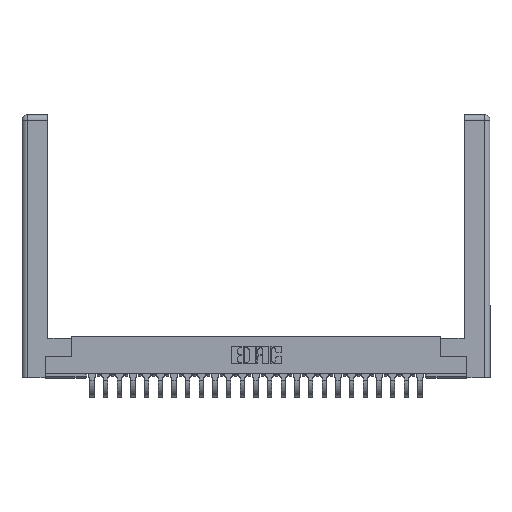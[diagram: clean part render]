
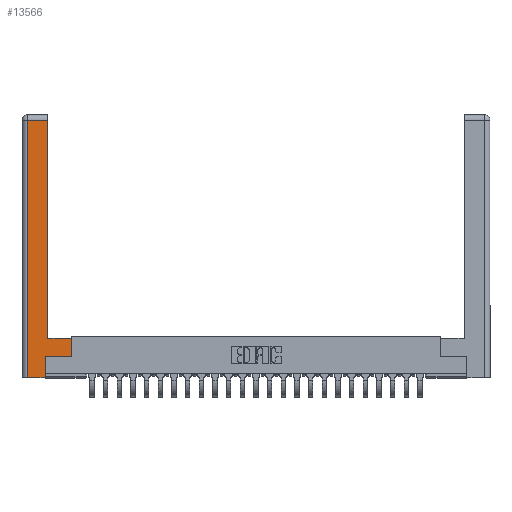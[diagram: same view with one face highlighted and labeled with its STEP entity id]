
A CAD part, top view. The second image highlights one B-rep face of the part: STEP entity #13566.
In plain terms, the highlighted planar face has unit normal (0, 0, 1).
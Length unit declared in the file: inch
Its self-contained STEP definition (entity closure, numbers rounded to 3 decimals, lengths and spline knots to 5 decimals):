
#136 = CARTESIAN_POINT ( 'NONE',  ( 0.295, 0.45, 0. ) ) ;
#204 = LINE ( 'NONE', #8691, #4602 ) ;
#393 = ORIENTED_EDGE ( 'NONE', *, *, #6340, .T. ) ;
#554 = CARTESIAN_POINT ( 'NONE',  ( 0.295, 2.94, 0. ) ) ;
#651 = VERTEX_POINT ( 'NONE', #9319 ) ;
#791 = LINE ( 'NONE', #5931, #28143 ) ;
#862 = LINE ( 'NONE', #2461, #1909 ) ;
#1330 = DIRECTION ( 'NONE',  ( 1., 0., 0. ) ) ;
#1909 = VECTOR ( 'NONE', #9493, 39.37008 ) ;
#1943 = CARTESIAN_POINT ( 'NONE',  ( 0.565, 0.245, 0. ) ) ;
#2307 = CARTESIAN_POINT ( 'NONE',  ( 0.0615, 0., 0. ) ) ;
#2461 = CARTESIAN_POINT ( 'NONE',  ( 0.0615, 2.94, 0. ) ) ;
#2630 = EDGE_CURVE ( 'NONE', #17095, #13198, #204, .T. ) ;
#3067 = CARTESIAN_POINT ( 'NONE',  ( 0.565, 0.45, 0. ) ) ;
#3112 = VERTEX_POINT ( 'NONE', #10985 ) ;
#3341 = LINE ( 'NONE', #3067, #16163 ) ;
#4367 = DIRECTION ( 'NONE',  ( 0., -1., 0. ) ) ;
#4386 = EDGE_CURVE ( 'NONE', #15528, #17095, #3341, .T. ) ;
#4602 = VECTOR ( 'NONE', #17358, 39.37008 ) ;
#5931 = CARTESIAN_POINT ( 'NONE',  ( 0.265, 0., 0. ) ) ;
#6170 = CARTESIAN_POINT ( 'NONE',  ( 0.565, 0.245, 0. ) ) ;
#6340 = EDGE_CURVE ( 'NONE', #13198, #10370, #17299, .T. ) ;
#7026 = VECTOR ( 'NONE', #15571, 39.37008 ) ;
#7243 = EDGE_CURVE ( 'NONE', #10370, #10028, #862, .T. ) ;
#7521 = ORIENTED_EDGE ( 'NONE', *, *, #2630, .T. ) ;
#7600 = AXIS2_PLACEMENT_3D ( 'NONE', #23996, #23858, #8455 ) ;
#8245 = EDGE_CURVE ( 'NONE', #27352, #651, #791, .T. ) ;
#8455 = DIRECTION ( 'NONE',  ( -1., 0., 0. ) ) ;
#8691 = CARTESIAN_POINT ( 'NONE',  ( 0.295, 0.45, 0. ) ) ;
#9319 = CARTESIAN_POINT ( 'NONE',  ( 0.265, 0., 0. ) ) ;
#9493 = DIRECTION ( 'NONE',  ( -1., 0., 0. ) ) ;
#9510 = LINE ( 'NONE', #6170, #9916 ) ;
#9916 = VECTOR ( 'NONE', #18323, 39.37008 ) ;
#10028 = VERTEX_POINT ( 'NONE', #18349 ) ;
#10370 = VERTEX_POINT ( 'NONE', #554 ) ;
#10666 = ORIENTED_EDGE ( 'NONE', *, *, #4386, .T. ) ;
#10985 = CARTESIAN_POINT ( 'NONE',  ( 0.265, 0.245, 0. ) ) ;
#11034 = PLANE ( 'NONE',  #7600 ) ;
#11095 = CARTESIAN_POINT ( 'NONE',  ( 0.265, 0.245, 0. ) ) ;
#11458 = ORIENTED_EDGE ( 'NONE', *, *, #7243, .T. ) ;
#11515 = ORIENTED_EDGE ( 'NONE', *, *, #11528, .T. ) ;
#11528 = EDGE_CURVE ( 'NONE', #651, #3112, #24479, .T. ) ;
#12132 = DIRECTION ( 'NONE',  ( 0., 1., 0. ) ) ;
#12236 = EDGE_LOOP ( 'NONE', ( #393, #11458, #26253, #17069, #11515, #17706, #10666, #7521 ) ) ;
#13198 = VERTEX_POINT ( 'NONE', #136 ) ;
#13432 = LINE ( 'NONE', #24087, #17399 ) ;
#13566 = ADVANCED_FACE ( 'NONE', ( #15086 ), #11034, .F. ) ;
#15086 = FACE_OUTER_BOUND ( 'NONE', #12236, .T. ) ;
#15528 = VERTEX_POINT ( 'NONE', #1943 ) ;
#15571 = DIRECTION ( 'NONE',  ( 0., 1., 0. ) ) ;
#16163 = VECTOR ( 'NONE', #12132, 39.37008 ) ;
#16775 = CARTESIAN_POINT ( 'NONE',  ( 0.565, 0.45, 0. ) ) ;
#16847 = VECTOR ( 'NONE', #23759, 39.37008 ) ;
#17069 = ORIENTED_EDGE ( 'NONE', *, *, #8245, .T. ) ;
#17095 = VERTEX_POINT ( 'NONE', #16775 ) ;
#17299 = LINE ( 'NONE', #27793, #16847 ) ;
#17358 = DIRECTION ( 'NONE',  ( -1., 0., 0. ) ) ;
#17399 = VECTOR ( 'NONE', #4367, 39.37008 ) ;
#17706 = ORIENTED_EDGE ( 'NONE', *, *, #24386, .T. ) ;
#18323 = DIRECTION ( 'NONE',  ( 1., 0., 0. ) ) ;
#18349 = CARTESIAN_POINT ( 'NONE',  ( 0.0615, 2.94, 0. ) ) ;
#18621 = EDGE_CURVE ( 'NONE', #10028, #27352, #13432, .T. ) ;
#23759 = DIRECTION ( 'NONE',  ( 0., 1., 0. ) ) ;
#23858 = DIRECTION ( 'NONE',  ( 0., 0., -1. ) ) ;
#23996 = CARTESIAN_POINT ( 'NONE',  ( 0., 0., 0. ) ) ;
#24087 = CARTESIAN_POINT ( 'NONE',  ( 0.0615, 0., 0. ) ) ;
#24386 = EDGE_CURVE ( 'NONE', #3112, #15528, #9510, .T. ) ;
#24479 = LINE ( 'NONE', #11095, #7026 ) ;
#26253 = ORIENTED_EDGE ( 'NONE', *, *, #18621, .T. ) ;
#27352 = VERTEX_POINT ( 'NONE', #2307 ) ;
#27793 = CARTESIAN_POINT ( 'NONE',  ( 0.295, 3., 0. ) ) ;
#28143 = VECTOR ( 'NONE', #1330, 39.37008 ) ;
